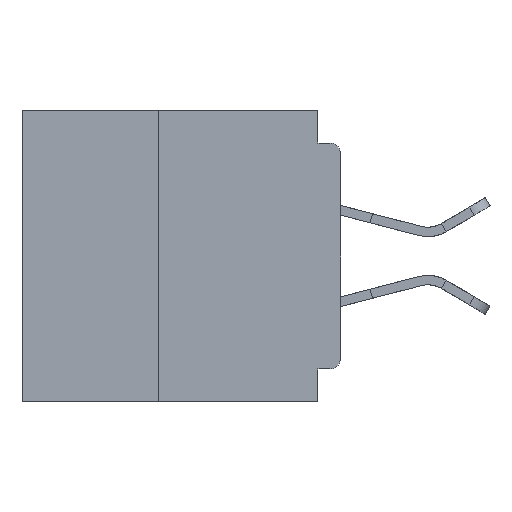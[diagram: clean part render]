
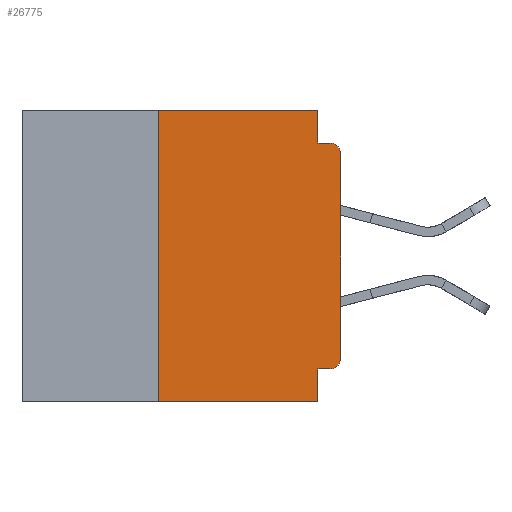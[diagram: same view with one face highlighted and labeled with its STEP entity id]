
A CAD part, left-side view. The second image highlights one B-rep face of the part: STEP entity #26775.
In plain terms, the highlighted planar face has unit normal (-1, 0, 0).
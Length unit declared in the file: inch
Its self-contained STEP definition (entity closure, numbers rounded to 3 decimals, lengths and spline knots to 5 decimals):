
#446 = DIRECTION ( 'NONE',  ( 0., 0., -1. ) ) ;
#919 = ORIENTED_EDGE ( 'NONE', *, *, #35701, .T. ) ;
#1320 = VECTOR ( 'NONE', #12706, 39.37008 ) ;
#1575 = DIRECTION ( 'NONE',  ( 0., 1., 0. ) ) ;
#1748 = VERTEX_POINT ( 'NONE', #12401 ) ;
#1792 = CARTESIAN_POINT ( 'NONE',  ( 0., 0., -0.06 ) ) ;
#2191 = LINE ( 'NONE', #17329, #41422 ) ;
#2301 = LINE ( 'NONE', #24577, #31438 ) ;
#2381 = ORIENTED_EDGE ( 'NONE', *, *, #15584, .F. ) ;
#3052 = LINE ( 'NONE', #11617, #32144 ) ;
#3876 = VERTEX_POINT ( 'NONE', #33404 ) ;
#5427 = CARTESIAN_POINT ( 'NONE',  ( 0., 0., -0.355 ) ) ;
#5673 = LINE ( 'NONE', #19134, #41317 ) ;
#7505 = ORIENTED_EDGE ( 'NONE', *, *, #11635, .F. ) ;
#8587 = VERTEX_POINT ( 'NONE', #41789 ) ;
#9473 = ORIENTED_EDGE ( 'NONE', *, *, #33540, .F. ) ;
#10246 = LINE ( 'NONE', #34208, #48226 ) ;
#11492 = DIRECTION ( 'NONE',  ( -1., 0., 0. ) ) ;
#11617 = CARTESIAN_POINT ( 'NONE',  ( 0., 0.437, 0. ) ) ;
#11635 = EDGE_CURVE ( 'NONE', #3876, #19980, #2301, .T. ) ;
#11735 = CARTESIAN_POINT ( 'NONE',  ( 0., 0.25, 0. ) ) ;
#12155 = VERTEX_POINT ( 'NONE', #12275 ) ;
#12258 = AXIS2_PLACEMENT_3D ( 'NONE', #19493, #23254, #446 ) ;
#12275 = CARTESIAN_POINT ( 'NONE',  ( 0., 0.25, -0.4 ) ) ;
#12401 = CARTESIAN_POINT ( 'NONE',  ( 0., 0.031, 0. ) ) ;
#12706 = DIRECTION ( 'NONE',  ( 0., -1., 0. ) ) ;
#13883 = ORIENTED_EDGE ( 'NONE', *, *, #34659, .F. ) ;
#14297 = CARTESIAN_POINT ( 'NONE',  ( 0., 0.015, -0.34 ) ) ;
#14430 = VERTEX_POINT ( 'NONE', #27334 ) ;
#14455 = LINE ( 'NONE', #5427, #33406 ) ;
#14712 = CARTESIAN_POINT ( 'NONE',  ( 0., 0.031, 0. ) ) ;
#15476 = DIRECTION ( 'NONE',  ( 0., -1., 0. ) ) ;
#15584 = EDGE_CURVE ( 'NONE', #12155, #47270, #5673, .T. ) ;
#17186 = ORIENTED_EDGE ( 'NONE', *, *, #46028, .T. ) ;
#17329 = CARTESIAN_POINT ( 'NONE',  ( 0., 0.437, -0.4 ) ) ;
#18131 = DIRECTION ( 'NONE',  ( 0., 0., -1. ) ) ;
#18778 = VECTOR ( 'NONE', #33568, 39.37008 ) ;
#19134 = CARTESIAN_POINT ( 'NONE',  ( 0., 0.25, -0.4 ) ) ;
#19154 = CIRCLE ( 'NONE', #36238, 0.015 ) ;
#19493 = CARTESIAN_POINT ( 'NONE',  ( 0., 0.437, 0. ) ) ;
#19620 = EDGE_LOOP ( 'NONE', ( #919, #17186, #35223, #9473, #46625, #2381, #41641, #7505, #13883, #36507 ) ) ;
#19980 = VERTEX_POINT ( 'NONE', #23438 ) ;
#22331 = CIRCLE ( 'NONE', #37175, 0.015 ) ;
#23002 = EDGE_CURVE ( 'NONE', #47270, #1748, #3052, .T. ) ;
#23254 = DIRECTION ( 'NONE',  ( 1., 0., 0. ) ) ;
#23438 = CARTESIAN_POINT ( 'NONE',  ( 0., 0.031, -0.4 ) ) ;
#24577 = CARTESIAN_POINT ( 'NONE',  ( 0., 0.031, -0.4 ) ) ;
#25870 = VERTEX_POINT ( 'NONE', #44571 ) ;
#26775 = ADVANCED_FACE ( 'NONE', ( #33416 ), #26928, .F. ) ;
#26928 = PLANE ( 'NONE',  #12258 ) ;
#27334 = CARTESIAN_POINT ( 'NONE',  ( 0., 0.031, -0.045 ) ) ;
#31438 = VECTOR ( 'NONE', #47302, 39.37008 ) ;
#31645 = LINE ( 'NONE', #43024, #1320 ) ;
#32144 = VECTOR ( 'NONE', #15476, 39.37008 ) ;
#32168 = EDGE_CURVE ( 'NONE', #12155, #19980, #2191, .T. ) ;
#32396 = CARTESIAN_POINT ( 'NONE',  ( 0., 0.015, -0.045 ) ) ;
#33404 = CARTESIAN_POINT ( 'NONE',  ( 0., 0.031, -0.355 ) ) ;
#33406 = VECTOR ( 'NONE', #1575, 39.37008 ) ;
#33416 = FACE_OUTER_BOUND ( 'NONE', #19620, .T. ) ;
#33540 = EDGE_CURVE ( 'NONE', #1748, #14430, #40091, .T. ) ;
#33568 = DIRECTION ( 'NONE',  ( 0., 0., -1. ) ) ;
#34202 = CARTESIAN_POINT ( 'NONE',  ( 0., 0.015, -0.06 ) ) ;
#34208 = CARTESIAN_POINT ( 'NONE',  ( 0., 0., 0. ) ) ;
#34659 = EDGE_CURVE ( 'NONE', #8587, #3876, #14455, .T. ) ;
#35223 = ORIENTED_EDGE ( 'NONE', *, *, #39252, .F. ) ;
#35701 = EDGE_CURVE ( 'NONE', #25870, #48163, #10246, .T. ) ;
#36165 = EDGE_CURVE ( 'NONE', #8587, #25870, #19154, .T. ) ;
#36238 = AXIS2_PLACEMENT_3D ( 'NONE', #14297, #40813, #18131 ) ;
#36507 = ORIENTED_EDGE ( 'NONE', *, *, #36165, .T. ) ;
#37175 = AXIS2_PLACEMENT_3D ( 'NONE', #34202, #11492, #38041 ) ;
#38041 = DIRECTION ( 'NONE',  ( 0., 0., -1. ) ) ;
#38048 = DIRECTION ( 'NONE',  ( 0., 0., 1. ) ) ;
#39252 = EDGE_CURVE ( 'NONE', #14430, #41137, #31645, .T. ) ;
#40091 = LINE ( 'NONE', #14712, #18778 ) ;
#40813 = DIRECTION ( 'NONE',  ( -1., 0., 0. ) ) ;
#41137 = VERTEX_POINT ( 'NONE', #32396 ) ;
#41317 = VECTOR ( 'NONE', #41812, 39.37008 ) ;
#41422 = VECTOR ( 'NONE', #47628, 39.37008 ) ;
#41641 = ORIENTED_EDGE ( 'NONE', *, *, #32168, .T. ) ;
#41789 = CARTESIAN_POINT ( 'NONE',  ( 0., 0.015, -0.355 ) ) ;
#41812 = DIRECTION ( 'NONE',  ( 0., 0., 1. ) ) ;
#43024 = CARTESIAN_POINT ( 'NONE',  ( 0., 0., -0.045 ) ) ;
#44571 = CARTESIAN_POINT ( 'NONE',  ( 0., 0., -0.34 ) ) ;
#46028 = EDGE_CURVE ( 'NONE', #48163, #41137, #22331, .T. ) ;
#46625 = ORIENTED_EDGE ( 'NONE', *, *, #23002, .F. ) ;
#47270 = VERTEX_POINT ( 'NONE', #11735 ) ;
#47302 = DIRECTION ( 'NONE',  ( 0., 0., -1. ) ) ;
#47628 = DIRECTION ( 'NONE',  ( 0., -1., 0. ) ) ;
#48163 = VERTEX_POINT ( 'NONE', #1792 ) ;
#48226 = VECTOR ( 'NONE', #38048, 39.37008 ) ;
